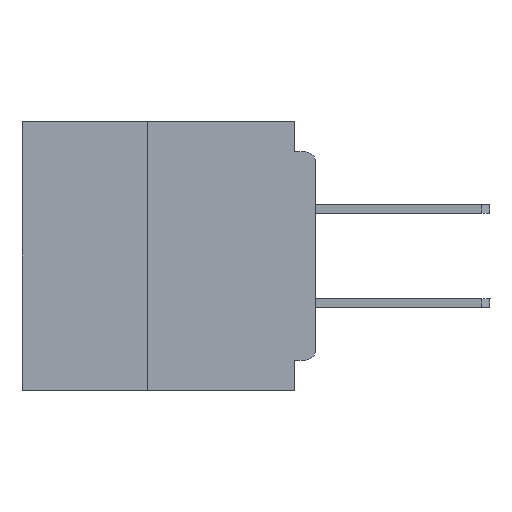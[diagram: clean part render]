
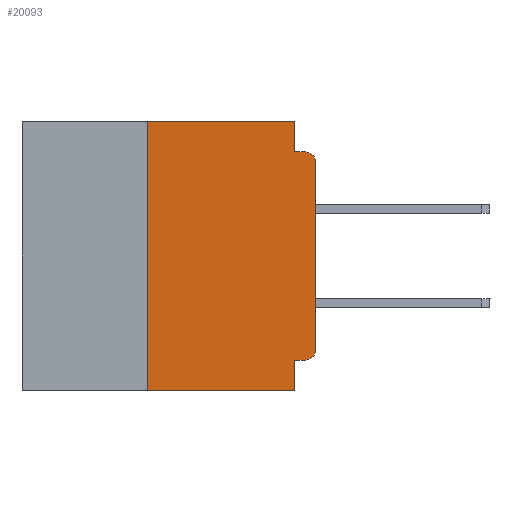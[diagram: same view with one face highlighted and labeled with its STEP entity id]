
A CAD part, left-side view. The second image highlights one B-rep face of the part: STEP entity #20093.
In plain terms, the highlighted planar face has unit normal (-1, 0, 0).
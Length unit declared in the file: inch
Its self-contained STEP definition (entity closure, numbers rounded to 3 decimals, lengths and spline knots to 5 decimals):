
#724 = EDGE_CURVE ( 'NONE', #22712, #55993, #6387, .T. ) ;
#1270 = ORIENTED_EDGE ( 'NONE', *, *, #35005, .F. ) ;
#1574 = CARTESIAN_POINT ( 'NONE',  ( 0., 0.015, -0.355 ) ) ;
#1625 = VERTEX_POINT ( 'NONE', #62037 ) ;
#1805 = EDGE_CURVE ( 'NONE', #1625, #10163, #36495, .T. ) ;
#4461 = EDGE_CURVE ( 'NONE', #5476, #36055, #49380, .T. ) ;
#5476 = VERTEX_POINT ( 'NONE', #1574 ) ;
#5787 = CARTESIAN_POINT ( 'NONE',  ( 0., 0., -0.045 ) ) ;
#6387 = CIRCLE ( 'NONE', #17443, 0.015 ) ;
#6563 = DIRECTION ( 'NONE',  ( 0., 0., -1. ) ) ;
#6593 = CARTESIAN_POINT ( 'NONE',  ( 0., 0.437, 0. ) ) ;
#6634 = CARTESIAN_POINT ( 'NONE',  ( 0., 0.031, 0. ) ) ;
#7228 = VERTEX_POINT ( 'NONE', #6634 ) ;
#7851 = CARTESIAN_POINT ( 'NONE',  ( 0., 0., 0. ) ) ;
#8486 = LINE ( 'NONE', #45555, #21705 ) ;
#9786 = EDGE_CURVE ( 'NONE', #7228, #34330, #19676, .T. ) ;
#9979 = CARTESIAN_POINT ( 'NONE',  ( 0., 0.031, -0.4 ) ) ;
#10163 = VERTEX_POINT ( 'NONE', #19213 ) ;
#10747 = FACE_OUTER_BOUND ( 'NONE', #48102, .T. ) ;
#10792 = DIRECTION ( 'NONE',  ( 0., -1., 0. ) ) ;
#11011 = DIRECTION ( 'NONE',  ( 0., 1., 0. ) ) ;
#11205 = ORIENTED_EDGE ( 'NONE', *, *, #35659, .F. ) ;
#11587 = DIRECTION ( 'NONE',  ( 0., -1., 0. ) ) ;
#12524 = DIRECTION ( 'NONE',  ( 1., 0., 0. ) ) ;
#13047 = DIRECTION ( 'NONE',  ( 0., 0., -1. ) ) ;
#13112 = DIRECTION ( 'NONE',  ( -1., 0., 0. ) ) ;
#13189 = CARTESIAN_POINT ( 'NONE',  ( 0., 0.015, -0.06 ) ) ;
#14408 = CARTESIAN_POINT ( 'NONE',  ( 0., 0.031, -0.045 ) ) ;
#16352 = CARTESIAN_POINT ( 'NONE',  ( 0., 0.031, 0. ) ) ;
#17443 = AXIS2_PLACEMENT_3D ( 'NONE', #13189, #13112, #13047 ) ;
#17887 = VECTOR ( 'NONE', #11587, 39.37008 ) ;
#18479 = LINE ( 'NONE', #5787, #43125 ) ;
#18657 = DIRECTION ( 'NONE',  ( -1., 0., 0. ) ) ;
#19213 = CARTESIAN_POINT ( 'NONE',  ( 0., 0.031, -0.4 ) ) ;
#19676 = LINE ( 'NONE', #16352, #44333 ) ;
#20093 = ADVANCED_FACE ( 'NONE', ( #10747 ), #56704, .F. ) ;
#20994 = DIRECTION ( 'NONE',  ( 0., 0., 1. ) ) ;
#21216 = CARTESIAN_POINT ( 'NONE',  ( 0., 0.031, -0.355 ) ) ;
#21705 = VECTOR ( 'NONE', #11011, 39.37008 ) ;
#21729 = ORIENTED_EDGE ( 'NONE', *, *, #25046, .T. ) ;
#22712 = VERTEX_POINT ( 'NONE', #35850 ) ;
#23727 = VECTOR ( 'NONE', #20994, 39.37008 ) ;
#25046 = EDGE_CURVE ( 'NONE', #36055, #22712, #57598, .T. ) ;
#26003 = ORIENTED_EDGE ( 'NONE', *, *, #1805, .T. ) ;
#29610 = CARTESIAN_POINT ( 'NONE',  ( 0., 0.25, 0. ) ) ;
#31453 = VECTOR ( 'NONE', #61847, 39.37008 ) ;
#31976 = ORIENTED_EDGE ( 'NONE', *, *, #49851, .F. ) ;
#32011 = CARTESIAN_POINT ( 'NONE',  ( 0., 0.437, 0. ) ) ;
#34330 = VERTEX_POINT ( 'NONE', #14408 ) ;
#34655 = DIRECTION ( 'NONE',  ( 0., 0., -1. ) ) ;
#34924 = VECTOR ( 'NONE', #43857, 39.37008 ) ;
#34927 = CARTESIAN_POINT ( 'NONE',  ( 0., 0.015, -0.045 ) ) ;
#35005 = EDGE_CURVE ( 'NONE', #59572, #10163, #62134, .T. ) ;
#35262 = LINE ( 'NONE', #50444, #23727 ) ;
#35659 = EDGE_CURVE ( 'NONE', #1625, #63573, #35262, .T. ) ;
#35771 = AXIS2_PLACEMENT_3D ( 'NONE', #48125, #18657, #53047 ) ;
#35850 = CARTESIAN_POINT ( 'NONE',  ( 0., 0., -0.06 ) ) ;
#36055 = VERTEX_POINT ( 'NONE', #48486 ) ;
#36136 = VECTOR ( 'NONE', #34655, 39.37008 ) ;
#36495 = LINE ( 'NONE', #38940, #34924 ) ;
#38940 = CARTESIAN_POINT ( 'NONE',  ( 0., 0.437, -0.4 ) ) ;
#40123 = AXIS2_PLACEMENT_3D ( 'NONE', #32011, #12524, #47065 ) ;
#43125 = VECTOR ( 'NONE', #10792, 39.37008 ) ;
#43857 = DIRECTION ( 'NONE',  ( 0., -1., 0. ) ) ;
#44324 = ORIENTED_EDGE ( 'NONE', *, *, #45604, .F. ) ;
#44333 = VECTOR ( 'NONE', #6563, 39.37008 ) ;
#45555 = CARTESIAN_POINT ( 'NONE',  ( 0., 0., -0.355 ) ) ;
#45604 = EDGE_CURVE ( 'NONE', #5476, #59572, #8486, .T. ) ;
#47065 = DIRECTION ( 'NONE',  ( 0., 0., -1. ) ) ;
#48102 = EDGE_LOOP ( 'NONE', ( #21729, #56689, #60366, #54517, #31976, #11205, #26003, #1270, #44324, #63175 ) ) ;
#48125 = CARTESIAN_POINT ( 'NONE',  ( 0., 0.015, -0.34 ) ) ;
#48486 = CARTESIAN_POINT ( 'NONE',  ( 0., 0., -0.34 ) ) ;
#49380 = CIRCLE ( 'NONE', #35771, 0.015 ) ;
#49851 = EDGE_CURVE ( 'NONE', #63573, #7228, #57131, .T. ) ;
#50444 = CARTESIAN_POINT ( 'NONE',  ( 0., 0.25, -0.4 ) ) ;
#53047 = DIRECTION ( 'NONE',  ( 0., 0., -1. ) ) ;
#54517 = ORIENTED_EDGE ( 'NONE', *, *, #9786, .F. ) ;
#55993 = VERTEX_POINT ( 'NONE', #34927 ) ;
#56689 = ORIENTED_EDGE ( 'NONE', *, *, #724, .T. ) ;
#56704 = PLANE ( 'NONE',  #40123 ) ;
#57131 = LINE ( 'NONE', #6593, #17887 ) ;
#57598 = LINE ( 'NONE', #7851, #31453 ) ;
#59572 = VERTEX_POINT ( 'NONE', #21216 ) ;
#60366 = ORIENTED_EDGE ( 'NONE', *, *, #63696, .F. ) ;
#61847 = DIRECTION ( 'NONE',  ( 0., 0., 1. ) ) ;
#62037 = CARTESIAN_POINT ( 'NONE',  ( 0., 0.25, -0.4 ) ) ;
#62134 = LINE ( 'NONE', #9979, #36136 ) ;
#63175 = ORIENTED_EDGE ( 'NONE', *, *, #4461, .T. ) ;
#63573 = VERTEX_POINT ( 'NONE', #29610 ) ;
#63696 = EDGE_CURVE ( 'NONE', #34330, #55993, #18479, .T. ) ;
